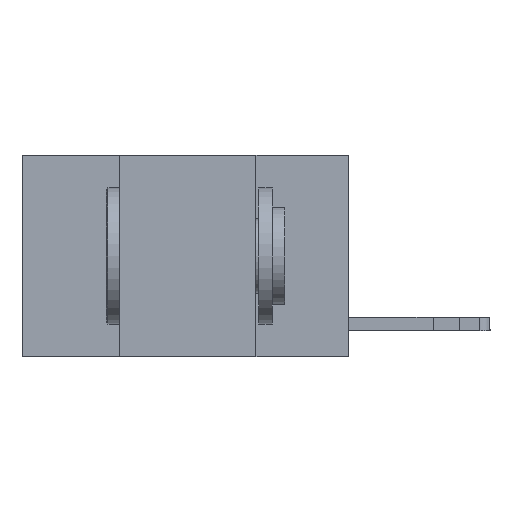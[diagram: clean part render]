
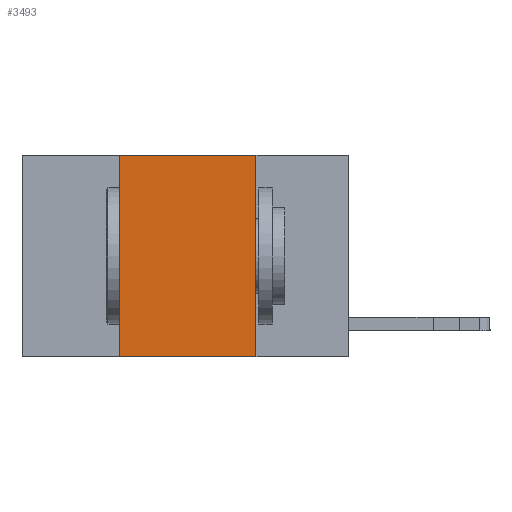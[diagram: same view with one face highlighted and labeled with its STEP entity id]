
A CAD part, left-side view. The second image highlights one B-rep face of the part: STEP entity #3493.
In plain terms, the highlighted planar face has unit normal (-1, 0, 0).
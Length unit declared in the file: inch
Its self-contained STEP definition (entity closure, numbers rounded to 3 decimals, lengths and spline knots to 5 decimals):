
#765 = CARTESIAN_POINT ( 'NONE',  ( 0., 0.6, -0.37 ) ) ;
#1086 = CARTESIAN_POINT ( 'NONE',  ( 0., 0.42, 0. ) ) ;
#2209 = VECTOR ( 'NONE', #3173, 39.37008 ) ;
#2294 = CARTESIAN_POINT ( 'NONE',  ( 0., 0.17, 0. ) ) ;
#2360 = EDGE_CURVE ( 'NONE', #5913, #11064, #3125, .T. ) ;
#3125 = LINE ( 'NONE', #12764, #5370 ) ;
#3129 = CARTESIAN_POINT ( 'NONE',  ( 0., 0.42, -0.37 ) ) ;
#3173 = DIRECTION ( 'NONE',  ( 0., -1., 0. ) ) ;
#3487 = DIRECTION ( 'NONE',  ( 0., 0., 1. ) ) ;
#3493 = ADVANCED_FACE ( 'NONE', ( #7189 ), #11989, .F. ) ;
#4338 = LINE ( 'NONE', #765, #2209 ) ;
#4811 = ORIENTED_EDGE ( 'NONE', *, *, #2360, .F. ) ;
#5033 = DIRECTION ( 'NONE',  ( 0., -1., 0. ) ) ;
#5035 = VERTEX_POINT ( 'NONE', #3129 ) ;
#5073 = EDGE_CURVE ( 'NONE', #8597, #5913, #6268, .T. ) ;
#5370 = VECTOR ( 'NONE', #7963, 39.37008 ) ;
#5685 = CARTESIAN_POINT ( 'NONE',  ( 0., 0.42, 0. ) ) ;
#5913 = VERTEX_POINT ( 'NONE', #2294 ) ;
#6195 = CARTESIAN_POINT ( 'NONE',  ( 0., 0.6, 0. ) ) ;
#6268 = LINE ( 'NONE', #6195, #9995 ) ;
#7189 = FACE_OUTER_BOUND ( 'NONE', #10955, .T. ) ;
#7491 = EDGE_CURVE ( 'NONE', #5035, #11064, #4338, .T. ) ;
#7963 = DIRECTION ( 'NONE',  ( 0., 0., -1. ) ) ;
#8172 = VECTOR ( 'NONE', #3487, 39.37008 ) ;
#8597 = VERTEX_POINT ( 'NONE', #1086 ) ;
#9542 = CARTESIAN_POINT ( 'NONE',  ( 0., 0.6, 0. ) ) ;
#9995 = VECTOR ( 'NONE', #5033, 39.37008 ) ;
#10061 = ORIENTED_EDGE ( 'NONE', *, *, #14179, .F. ) ;
#10697 = LINE ( 'NONE', #5685, #8172 ) ;
#10955 = EDGE_LOOP ( 'NONE', ( #4811, #13633, #10061, #15058 ) ) ;
#11044 = CARTESIAN_POINT ( 'NONE',  ( 0., 0.17, -0.37 ) ) ;
#11064 = VERTEX_POINT ( 'NONE', #11044 ) ;
#11695 = AXIS2_PLACEMENT_3D ( 'NONE', #9542, #14331, #12144 ) ;
#11989 = PLANE ( 'NONE',  #11695 ) ;
#12144 = DIRECTION ( 'NONE',  ( 0., 0., -1. ) ) ;
#12764 = CARTESIAN_POINT ( 'NONE',  ( 0., 0.17, 0. ) ) ;
#13633 = ORIENTED_EDGE ( 'NONE', *, *, #5073, .F. ) ;
#14179 = EDGE_CURVE ( 'NONE', #5035, #8597, #10697, .T. ) ;
#14331 = DIRECTION ( 'NONE',  ( 1., 0., 0. ) ) ;
#15058 = ORIENTED_EDGE ( 'NONE', *, *, #7491, .T. ) ;
